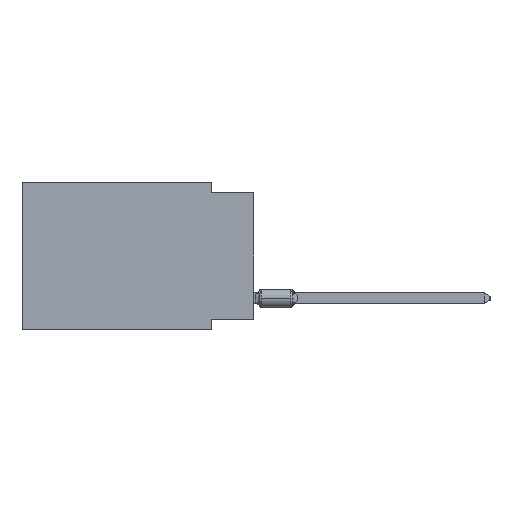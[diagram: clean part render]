
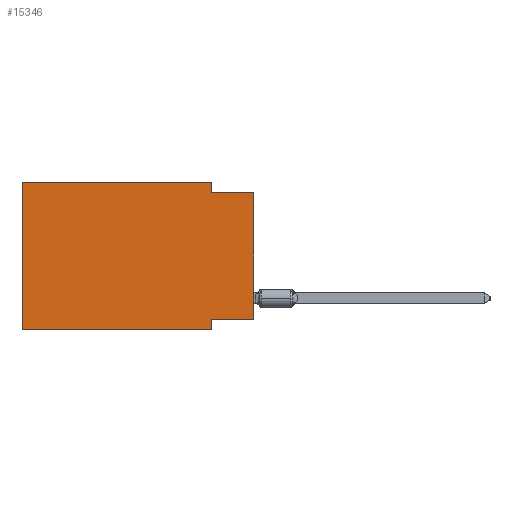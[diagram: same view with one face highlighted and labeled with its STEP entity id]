
A CAD part, left-side view. The second image highlights one B-rep face of the part: STEP entity #15346.
In plain terms, the highlighted planar face has unit normal (-1, 0, 0).
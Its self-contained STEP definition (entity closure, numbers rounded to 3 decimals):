
#350 = CARTESIAN_POINT ( 'NONE',  ( 0., 0., 0. ) ) ;
#568 = PLANE ( 'NONE',  #2380 ) ;
#1190 = LINE ( 'NONE', #23821, #26428 ) ;
#2380 = AXIS2_PLACEMENT_3D ( 'NONE', #16455, #25495, #4671 ) ;
#2882 = VECTOR ( 'NONE', #50756, 1000. ) ;
#3267 = CARTESIAN_POINT ( 'NONE',  ( 0., 2.54, -0.635 ) ) ;
#4397 = FACE_OUTER_BOUND ( 'NONE', #44657, .T. ) ;
#4474 = DIRECTION ( 'NONE',  ( 0., -1., 0. ) ) ;
#4671 = DIRECTION ( 'NONE',  ( 0., 0., -1. ) ) ;
#5556 = CARTESIAN_POINT ( 'NONE',  ( 0., 13.97, -8.89 ) ) ;
#6522 = EDGE_CURVE ( 'NONE', #42001, #31058, #26704, .T. ) ;
#7825 = LINE ( 'NONE', #49748, #33731 ) ;
#10884 = EDGE_CURVE ( 'NONE', #42001, #46645, #34066, .T. ) ;
#11212 = LINE ( 'NONE', #23299, #45280 ) ;
#11465 = LINE ( 'NONE', #37976, #43399 ) ;
#11517 = EDGE_CURVE ( 'NONE', #31058, #19080, #11465, .T. ) ;
#11918 = CARTESIAN_POINT ( 'NONE',  ( 0., 0., -8.255 ) ) ;
#12169 = VERTEX_POINT ( 'NONE', #11918 ) ;
#13349 = EDGE_CURVE ( 'NONE', #47877, #47778, #7825, .T. ) ;
#15346 = ADVANCED_FACE ( 'NONE', ( #4397 ), #568, .F. ) ;
#16455 = CARTESIAN_POINT ( 'NONE',  ( 0., 13.97, 0. ) ) ;
#16709 = CARTESIAN_POINT ( 'NONE',  ( 0., 2.54, -8.255 ) ) ;
#16872 = DIRECTION ( 'NONE',  ( 0., -1., 0. ) ) ;
#17748 = CARTESIAN_POINT ( 'NONE',  ( 0., 13.97, -8.89 ) ) ;
#18207 = DIRECTION ( 'NONE',  ( 0., 0., 1. ) ) ;
#19080 = VERTEX_POINT ( 'NONE', #26468 ) ;
#19528 = ORIENTED_EDGE ( 'NONE', *, *, #46042, .F. ) ;
#20067 = ORIENTED_EDGE ( 'NONE', *, *, #23295, .T. ) ;
#23294 = DIRECTION ( 'NONE',  ( 0., 1., 0. ) ) ;
#23295 = EDGE_CURVE ( 'NONE', #12169, #47778, #46110, .T. ) ;
#23299 = CARTESIAN_POINT ( 'NONE',  ( 0., 2.54, -8.89 ) ) ;
#23500 = ORIENTED_EDGE ( 'NONE', *, *, #35355, .F. ) ;
#23821 = CARTESIAN_POINT ( 'NONE',  ( 0., 0., -8.255 ) ) ;
#24909 = ORIENTED_EDGE ( 'NONE', *, *, #6522, .F. ) ;
#25495 = DIRECTION ( 'NONE',  ( 1., 0., 0. ) ) ;
#25662 = EDGE_CURVE ( 'NONE', #19080, #47877, #31285, .T. ) ;
#26428 = VECTOR ( 'NONE', #23294, 1000. ) ;
#26468 = CARTESIAN_POINT ( 'NONE',  ( 0., 2.54, 0. ) ) ;
#26704 = LINE ( 'NONE', #39306, #41241 ) ;
#27197 = CARTESIAN_POINT ( 'NONE',  ( 0., 13.97, 0. ) ) ;
#28206 = CARTESIAN_POINT ( 'NONE',  ( 0., 0., -0.635 ) ) ;
#31058 = VERTEX_POINT ( 'NONE', #27197 ) ;
#31285 = LINE ( 'NONE', #48012, #38832 ) ;
#31446 = ORIENTED_EDGE ( 'NONE', *, *, #13349, .F. ) ;
#33731 = VECTOR ( 'NONE', #16872, 1000. ) ;
#34066 = LINE ( 'NONE', #5556, #36333 ) ;
#35355 = EDGE_CURVE ( 'NONE', #50191, #46645, #11212, .T. ) ;
#36333 = VECTOR ( 'NONE', #4474, 1000. ) ;
#37976 = CARTESIAN_POINT ( 'NONE',  ( 0., 13.97, 0. ) ) ;
#38832 = VECTOR ( 'NONE', #44174, 1000. ) ;
#39306 = CARTESIAN_POINT ( 'NONE',  ( 0., 13.97, 0. ) ) ;
#41241 = VECTOR ( 'NONE', #18207, 1000. ) ;
#42001 = VERTEX_POINT ( 'NONE', #17748 ) ;
#42060 = ORIENTED_EDGE ( 'NONE', *, *, #10884, .T. ) ;
#43399 = VECTOR ( 'NONE', #52853, 1000. ) ;
#44174 = DIRECTION ( 'NONE',  ( 0., 0., -1. ) ) ;
#44657 = EDGE_LOOP ( 'NONE', ( #20067, #31446, #48893, #52543, #24909, #42060, #23500, #19528 ) ) ;
#45280 = VECTOR ( 'NONE', #52332, 1000. ) ;
#46042 = EDGE_CURVE ( 'NONE', #12169, #50191, #1190, .T. ) ;
#46110 = LINE ( 'NONE', #350, #2882 ) ;
#46645 = VERTEX_POINT ( 'NONE', #53877 ) ;
#47778 = VERTEX_POINT ( 'NONE', #28206 ) ;
#47877 = VERTEX_POINT ( 'NONE', #3267 ) ;
#48012 = CARTESIAN_POINT ( 'NONE',  ( 0., 2.54, 0. ) ) ;
#48893 = ORIENTED_EDGE ( 'NONE', *, *, #25662, .F. ) ;
#49748 = CARTESIAN_POINT ( 'NONE',  ( 0., 0., -0.635 ) ) ;
#50191 = VERTEX_POINT ( 'NONE', #16709 ) ;
#50756 = DIRECTION ( 'NONE',  ( 0., 0., 1. ) ) ;
#52332 = DIRECTION ( 'NONE',  ( 0., 0., -1. ) ) ;
#52543 = ORIENTED_EDGE ( 'NONE', *, *, #11517, .F. ) ;
#52853 = DIRECTION ( 'NONE',  ( 0., -1., 0. ) ) ;
#53877 = CARTESIAN_POINT ( 'NONE',  ( 0., 2.54, -8.89 ) ) ;
